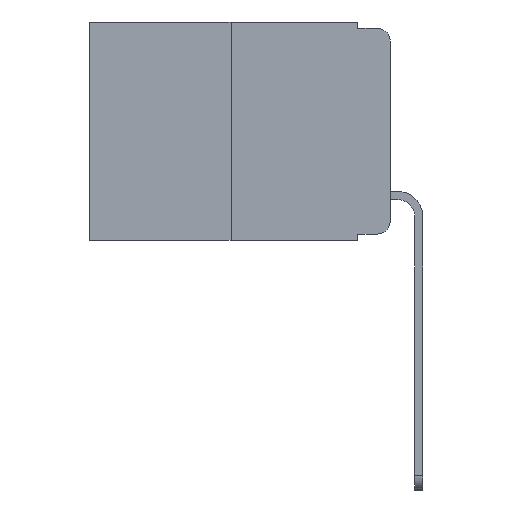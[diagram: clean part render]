
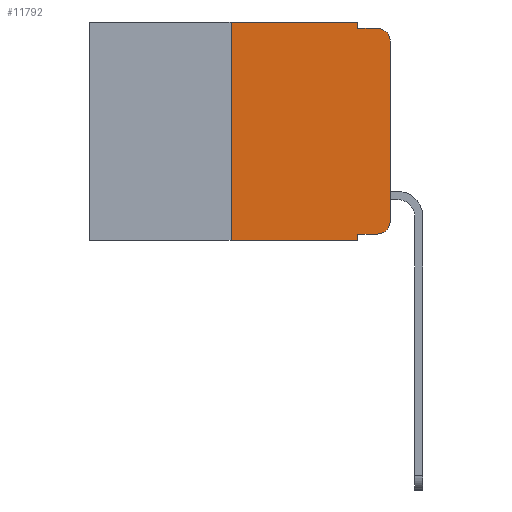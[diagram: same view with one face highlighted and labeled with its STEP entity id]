
A CAD part, left-side view. The second image highlights one B-rep face of the part: STEP entity #11792.
In plain terms, the highlighted planar face has unit normal (-1, 0, 0).
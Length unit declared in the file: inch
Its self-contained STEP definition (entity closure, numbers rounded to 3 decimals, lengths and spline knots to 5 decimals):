
#326 = ORIENTED_EDGE ( 'NONE', *, *, #11938, .T. ) ;
#518 = VERTEX_POINT ( 'NONE', #4898 ) ;
#542 = CARTESIAN_POINT ( 'NONE',  ( 0., 0.051, -0.333 ) ) ;
#626 = VECTOR ( 'NONE', #5850, 39.37008 ) ;
#790 = EDGE_LOOP ( 'NONE', ( #1195, #12301, #7404, #12980, #5671, #11170, #326, #11833, #6595, #12142 ) ) ;
#1065 = DIRECTION ( 'NONE',  ( -1., 0., 0. ) ) ;
#1195 = ORIENTED_EDGE ( 'NONE', *, *, #9862, .T. ) ;
#1365 = CARTESIAN_POINT ( 'NONE',  ( 0., 0.25, 0. ) ) ;
#1513 = DIRECTION ( 'NONE',  ( -1., 0., 0. ) ) ;
#1780 = CARTESIAN_POINT ( 'NONE',  ( 0., 0.02, -0.01 ) ) ;
#2238 = AXIS2_PLACEMENT_3D ( 'NONE', #7335, #1065, #8396 ) ;
#2455 = EDGE_CURVE ( 'NONE', #2475, #4041, #7823, .T. ) ;
#2475 = VERTEX_POINT ( 'NONE', #5278 ) ;
#3001 = VERTEX_POINT ( 'NONE', #6259 ) ;
#3044 = EDGE_CURVE ( 'NONE', #6489, #2475, #9324, .T. ) ;
#3047 = CIRCLE ( 'NONE', #11823, 0.02 ) ;
#3065 = LINE ( 'NONE', #12438, #4852 ) ;
#3104 = DIRECTION ( 'NONE',  ( 0., 0., -1. ) ) ;
#3308 = CARTESIAN_POINT ( 'NONE',  ( 0., 0.473, 0. ) ) ;
#3481 = CARTESIAN_POINT ( 'NONE',  ( 0., 0., 0. ) ) ;
#3732 = FACE_OUTER_BOUND ( 'NONE', #790, .T. ) ;
#4041 = VERTEX_POINT ( 'NONE', #11119 ) ;
#4491 = DIRECTION ( 'NONE',  ( 0., 0., 1. ) ) ;
#4601 = DIRECTION ( 'NONE',  ( 0., 0., 1. ) ) ;
#4807 = CARTESIAN_POINT ( 'NONE',  ( 0., 0.051, -0.01 ) ) ;
#4843 = LINE ( 'NONE', #7393, #12786 ) ;
#4852 = VECTOR ( 'NONE', #13489, 39.37008 ) ;
#4898 = CARTESIAN_POINT ( 'NONE',  ( 0., 0.051, -0.343 ) ) ;
#5278 = CARTESIAN_POINT ( 'NONE',  ( 0., 0.051, 0. ) ) ;
#5671 = ORIENTED_EDGE ( 'NONE', *, *, #3044, .F. ) ;
#5850 = DIRECTION ( 'NONE',  ( 0., -1., 0. ) ) ;
#5909 = EDGE_CURVE ( 'NONE', #4041, #7445, #10092, .T. ) ;
#6259 = CARTESIAN_POINT ( 'NONE',  ( 0., 0.02, -0.333 ) ) ;
#6489 = VERTEX_POINT ( 'NONE', #9549 ) ;
#6595 = ORIENTED_EDGE ( 'NONE', *, *, #11599, .T. ) ;
#6827 = CARTESIAN_POINT ( 'NONE',  ( 0., 0.25, -0.343 ) ) ;
#6997 = VERTEX_POINT ( 'NONE', #10327 ) ;
#7260 = DIRECTION ( 'NONE',  ( 0., 0., -1. ) ) ;
#7335 = CARTESIAN_POINT ( 'NONE',  ( 0., 0.02, -0.313 ) ) ;
#7346 = DIRECTION ( 'NONE',  ( 0., -1., 0. ) ) ;
#7393 = CARTESIAN_POINT ( 'NONE',  ( 0., 0.473, -0.343 ) ) ;
#7404 = ORIENTED_EDGE ( 'NONE', *, *, #5909, .F. ) ;
#7445 = VERTEX_POINT ( 'NONE', #1780 ) ;
#7646 = EDGE_CURVE ( 'NONE', #3001, #10049, #12473, .T. ) ;
#7731 = CARTESIAN_POINT ( 'NONE',  ( 0., 0.02, -0.03 ) ) ;
#7823 = LINE ( 'NONE', #12480, #10296 ) ;
#8224 = EDGE_CURVE ( 'NONE', #13505, #6489, #9553, .T. ) ;
#8396 = DIRECTION ( 'NONE',  ( 0., 0., -1. ) ) ;
#8594 = VERTEX_POINT ( 'NONE', #11737 ) ;
#8654 = VECTOR ( 'NONE', #7346, 39.37008 ) ;
#8694 = EDGE_CURVE ( 'NONE', #8594, #7445, #3047, .T. ) ;
#8710 = LINE ( 'NONE', #542, #626 ) ;
#8812 = DIRECTION ( 'NONE',  ( 0., 0., -1. ) ) ;
#9148 = AXIS2_PLACEMENT_3D ( 'NONE', #12376, #9306, #3104 ) ;
#9259 = PLANE ( 'NONE',  #9148 ) ;
#9306 = DIRECTION ( 'NONE',  ( 1., 0., 0. ) ) ;
#9324 = LINE ( 'NONE', #3308, #8654 ) ;
#9549 = CARTESIAN_POINT ( 'NONE',  ( 0., 0.25, 0. ) ) ;
#9553 = LINE ( 'NONE', #1365, #11965 ) ;
#9796 = VECTOR ( 'NONE', #10981, 39.37008 ) ;
#9862 = EDGE_CURVE ( 'NONE', #10049, #8594, #10457, .T. ) ;
#10049 = VERTEX_POINT ( 'NONE', #11044 ) ;
#10092 = LINE ( 'NONE', #4807, #9796 ) ;
#10296 = VECTOR ( 'NONE', #7260, 39.37008 ) ;
#10327 = CARTESIAN_POINT ( 'NONE',  ( 0., 0.051, -0.333 ) ) ;
#10457 = LINE ( 'NONE', #3481, #13225 ) ;
#10747 = EDGE_CURVE ( 'NONE', #6997, #518, #3065, .T. ) ;
#10981 = DIRECTION ( 'NONE',  ( 0., -1., 0. ) ) ;
#11044 = CARTESIAN_POINT ( 'NONE',  ( 0., 0., -0.313 ) ) ;
#11119 = CARTESIAN_POINT ( 'NONE',  ( 0., 0.051, -0.01 ) ) ;
#11170 = ORIENTED_EDGE ( 'NONE', *, *, #8224, .F. ) ;
#11599 = EDGE_CURVE ( 'NONE', #6997, #3001, #8710, .T. ) ;
#11737 = CARTESIAN_POINT ( 'NONE',  ( 0., 0., -0.03 ) ) ;
#11792 = ADVANCED_FACE ( 'NONE', ( #3732 ), #9259, .F. ) ;
#11823 = AXIS2_PLACEMENT_3D ( 'NONE', #7731, #1513, #8812 ) ;
#11833 = ORIENTED_EDGE ( 'NONE', *, *, #10747, .F. ) ;
#11938 = EDGE_CURVE ( 'NONE', #13505, #518, #4843, .T. ) ;
#11965 = VECTOR ( 'NONE', #4601, 39.37008 ) ;
#12142 = ORIENTED_EDGE ( 'NONE', *, *, #7646, .T. ) ;
#12301 = ORIENTED_EDGE ( 'NONE', *, *, #8694, .T. ) ;
#12376 = CARTESIAN_POINT ( 'NONE',  ( 0., 0.473, 0. ) ) ;
#12438 = CARTESIAN_POINT ( 'NONE',  ( 0., 0.051, 0. ) ) ;
#12473 = CIRCLE ( 'NONE', #2238, 0.02 ) ;
#12480 = CARTESIAN_POINT ( 'NONE',  ( 0., 0.051, 0. ) ) ;
#12608 = DIRECTION ( 'NONE',  ( 0., -1., 0. ) ) ;
#12786 = VECTOR ( 'NONE', #12608, 39.37008 ) ;
#12980 = ORIENTED_EDGE ( 'NONE', *, *, #2455, .F. ) ;
#13225 = VECTOR ( 'NONE', #4491, 39.37008 ) ;
#13489 = DIRECTION ( 'NONE',  ( 0., 0., -1. ) ) ;
#13505 = VERTEX_POINT ( 'NONE', #6827 ) ;
